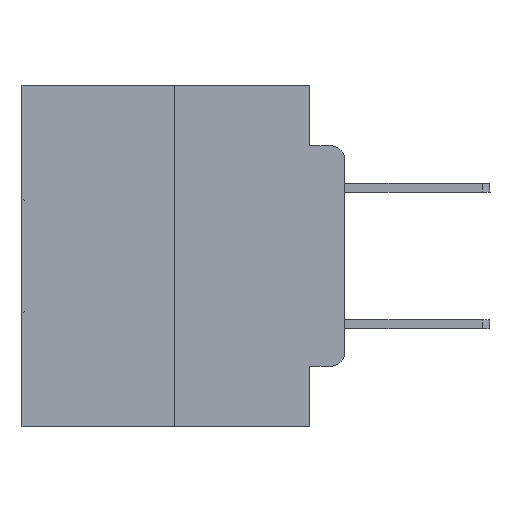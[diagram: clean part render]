
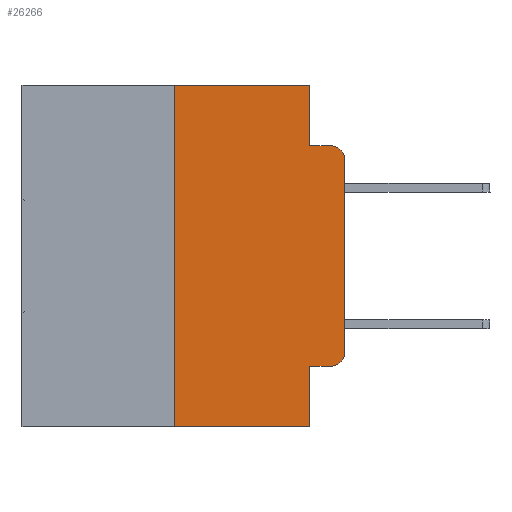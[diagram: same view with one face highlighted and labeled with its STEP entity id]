
A CAD part, left-side view. The second image highlights one B-rep face of the part: STEP entity #26266.
In plain terms, the highlighted planar face has unit normal (-1, 0, 0).
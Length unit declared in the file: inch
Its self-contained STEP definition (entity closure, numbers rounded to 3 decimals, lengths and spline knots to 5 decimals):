
#302 = DIRECTION ( 'NONE',  ( 0., 0., -1. ) ) ;
#2250 = DIRECTION ( 'NONE',  ( -1., 0., 0. ) ) ;
#2411 = VERTEX_POINT ( 'NONE', #30002 ) ;
#2711 = DIRECTION ( 'NONE',  ( 0., -1., 0. ) ) ;
#2747 = AXIS2_PLACEMENT_3D ( 'NONE', #10514, #5793, #22253 ) ;
#3863 = CARTESIAN_POINT ( 'NONE',  ( 0., 0.051, 0. ) ) ;
#4580 = ORIENTED_EDGE ( 'NONE', *, *, #20365, .F. ) ;
#4810 = LINE ( 'NONE', #10491, #22841 ) ;
#4930 = EDGE_CURVE ( 'NONE', #28450, #11188, #4810, .T. ) ;
#5491 = LINE ( 'NONE', #30393, #23531 ) ;
#5793 = DIRECTION ( 'NONE',  ( 1., 0., 0. ) ) ;
#6409 = AXIS2_PLACEMENT_3D ( 'NONE', #16427, #2250, #18789 ) ;
#6521 = EDGE_CURVE ( 'NONE', #28450, #28318, #28545, .T. ) ;
#6789 = ORIENTED_EDGE ( 'NONE', *, *, #4930, .T. ) ;
#7903 = ORIENTED_EDGE ( 'NONE', *, *, #25418, .T. ) ;
#8128 = EDGE_CURVE ( 'NONE', #24607, #23791, #15355, .T. ) ;
#8309 = ORIENTED_EDGE ( 'NONE', *, *, #29070, .T. ) ;
#8738 = DIRECTION ( 'NONE',  ( 0., -1., 0. ) ) ;
#9131 = VECTOR ( 'NONE', #13148, 39.37008 ) ;
#9261 = CARTESIAN_POINT ( 'NONE',  ( 0., 0., -0.3915 ) ) ;
#9430 = ORIENTED_EDGE ( 'NONE', *, *, #19170, .F. ) ;
#9936 = VECTOR ( 'NONE', #11846, 39.37008 ) ;
#9967 = CARTESIAN_POINT ( 'NONE',  ( 0., 0.051, -0.0885 ) ) ;
#10218 = CARTESIAN_POINT ( 'NONE',  ( 0., 0.02, -0.0885 ) ) ;
#10491 = CARTESIAN_POINT ( 'NONE',  ( 0., 0.051, -0.4115 ) ) ;
#10514 = CARTESIAN_POINT ( 'NONE',  ( 0., 0.473, 0. ) ) ;
#10595 = DIRECTION ( 'NONE',  ( 0., -1., 0. ) ) ;
#11188 = VERTEX_POINT ( 'NONE', #17172 ) ;
#11656 = ORIENTED_EDGE ( 'NONE', *, *, #28896, .T. ) ;
#11846 = DIRECTION ( 'NONE',  ( 0., 0., -1. ) ) ;
#12106 = CARTESIAN_POINT ( 'NONE',  ( 0., 0.25, -0.5 ) ) ;
#12258 = VECTOR ( 'NONE', #2711, 39.37008 ) ;
#12593 = VERTEX_POINT ( 'NONE', #15904 ) ;
#13148 = DIRECTION ( 'NONE',  ( 0., 0., 1. ) ) ;
#13562 = CARTESIAN_POINT ( 'NONE',  ( 0., 0.25, 0. ) ) ;
#13886 = CIRCLE ( 'NONE', #28307, 0.02 ) ;
#14313 = CARTESIAN_POINT ( 'NONE',  ( 0., 0.051, -0.4115 ) ) ;
#14518 = DIRECTION ( 'NONE',  ( -1., 0., 0. ) ) ;
#15355 = LINE ( 'NONE', #27071, #9131 ) ;
#15904 = CARTESIAN_POINT ( 'NONE',  ( 0., 0., -0.1085 ) ) ;
#16427 = CARTESIAN_POINT ( 'NONE',  ( 0., 0.02, -0.3915 ) ) ;
#16488 = DIRECTION ( 'NONE',  ( 0., -1., 0. ) ) ;
#17172 = CARTESIAN_POINT ( 'NONE',  ( 0., 0.02, -0.4115 ) ) ;
#17540 = PLANE ( 'NONE',  #2747 ) ;
#17570 = EDGE_CURVE ( 'NONE', #2411, #26770, #24735, .T. ) ;
#17624 = LINE ( 'NONE', #22784, #29259 ) ;
#18480 = LINE ( 'NONE', #21480, #12258 ) ;
#18726 = CIRCLE ( 'NONE', #6409, 0.02 ) ;
#18789 = DIRECTION ( 'NONE',  ( 0., 0., -1. ) ) ;
#19170 = EDGE_CURVE ( 'NONE', #26770, #19246, #18480, .T. ) ;
#19246 = VERTEX_POINT ( 'NONE', #10218 ) ;
#19645 = VERTEX_POINT ( 'NONE', #9261 ) ;
#20365 = EDGE_CURVE ( 'NONE', #23791, #2411, #5491, .T. ) ;
#21480 = CARTESIAN_POINT ( 'NONE',  ( 0., 0.051, -0.0885 ) ) ;
#21857 = ORIENTED_EDGE ( 'NONE', *, *, #17570, .F. ) ;
#22253 = DIRECTION ( 'NONE',  ( 0., 0., -1. ) ) ;
#22319 = DIRECTION ( 'NONE',  ( 0., 0., 1. ) ) ;
#22420 = CARTESIAN_POINT ( 'NONE',  ( 0., 0., 0. ) ) ;
#22701 = DIRECTION ( 'NONE',  ( 0., 0., -1. ) ) ;
#22784 = CARTESIAN_POINT ( 'NONE',  ( 0., 0.473, -0.5 ) ) ;
#22841 = VECTOR ( 'NONE', #10595, 39.37008 ) ;
#23353 = ORIENTED_EDGE ( 'NONE', *, *, #8128, .F. ) ;
#23531 = VECTOR ( 'NONE', #16488, 39.37008 ) ;
#23791 = VERTEX_POINT ( 'NONE', #13562 ) ;
#24607 = VERTEX_POINT ( 'NONE', #12106 ) ;
#24735 = LINE ( 'NONE', #3863, #30155 ) ;
#24803 = ORIENTED_EDGE ( 'NONE', *, *, #6521, .F. ) ;
#25418 = EDGE_CURVE ( 'NONE', #12593, #19246, #13886, .T. ) ;
#25539 = EDGE_LOOP ( 'NONE', ( #25908, #7903, #9430, #21857, #4580, #23353, #11656, #24803, #6789, #8309 ) ) ;
#25908 = ORIENTED_EDGE ( 'NONE', *, *, #26991, .T. ) ;
#26266 = ADVANCED_FACE ( 'NONE', ( #26698 ), #17540, .F. ) ;
#26498 = VECTOR ( 'NONE', #22319, 39.37008 ) ;
#26698 = FACE_OUTER_BOUND ( 'NONE', #25539, .T. ) ;
#26770 = VERTEX_POINT ( 'NONE', #9967 ) ;
#26991 = EDGE_CURVE ( 'NONE', #19645, #12593, #27223, .T. ) ;
#27071 = CARTESIAN_POINT ( 'NONE',  ( 0., 0.25, 0. ) ) ;
#27223 = LINE ( 'NONE', #22420, #26498 ) ;
#28155 = CARTESIAN_POINT ( 'NONE',  ( 0., 0.051, 0. ) ) ;
#28307 = AXIS2_PLACEMENT_3D ( 'NONE', #28487, #14518, #302 ) ;
#28318 = VERTEX_POINT ( 'NONE', #29993 ) ;
#28450 = VERTEX_POINT ( 'NONE', #14313 ) ;
#28487 = CARTESIAN_POINT ( 'NONE',  ( 0., 0.02, -0.1085 ) ) ;
#28545 = LINE ( 'NONE', #28155, #9936 ) ;
#28896 = EDGE_CURVE ( 'NONE', #24607, #28318, #17624, .T. ) ;
#29070 = EDGE_CURVE ( 'NONE', #11188, #19645, #18726, .T. ) ;
#29259 = VECTOR ( 'NONE', #8738, 39.37008 ) ;
#29993 = CARTESIAN_POINT ( 'NONE',  ( 0., 0.051, -0.5 ) ) ;
#30002 = CARTESIAN_POINT ( 'NONE',  ( 0., 0.051, 0. ) ) ;
#30155 = VECTOR ( 'NONE', #22701, 39.37008 ) ;
#30393 = CARTESIAN_POINT ( 'NONE',  ( 0., 0.473, 0. ) ) ;
